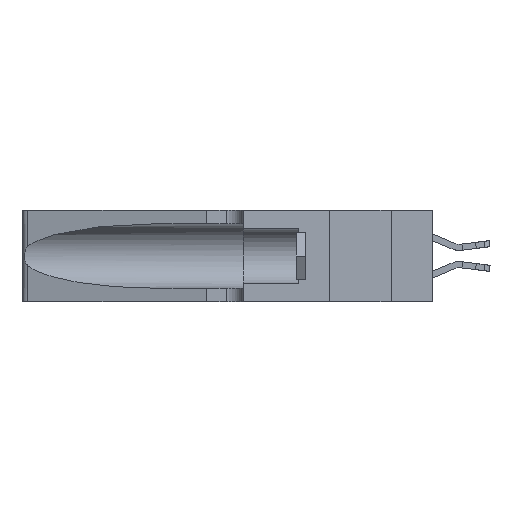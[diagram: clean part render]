
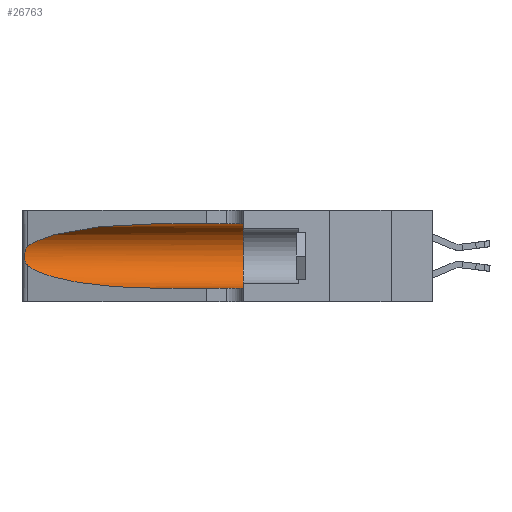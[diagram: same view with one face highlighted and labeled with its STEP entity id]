
A CAD part, left-side view. The second image highlights one B-rep face of the part: STEP entity #26763.
In plain terms, the highlighted cylindrical face has radius 3.308 mm (diameter 6.617 mm), a partial arc.
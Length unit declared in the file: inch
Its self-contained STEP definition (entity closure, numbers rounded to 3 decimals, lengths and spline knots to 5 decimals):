
#620 = ORIENTED_EDGE ( 'NONE', *, *, #31915, .T. ) ;
#2100 = AXIS2_PLACEMENT_3D ( 'NONE', #21576, #31954, #15879 ) ;
#2142 = CARTESIAN_POINT ( 'NONE',  ( 0.1305, 1.61858, 0.05475 ) ) ;
#2274 = CARTESIAN_POINT ( 'NONE',  ( 0.25487, 1.22718, 0.22369 ) ) ;
#3947 = ORIENTED_EDGE ( 'NONE', *, *, #4790, .T. ) ;
#4188 = VERTEX_POINT ( 'NONE', #12258 ) ;
#4305 = CARTESIAN_POINT ( 'NONE',  ( 0.25487, 1.22718, 0.22369 ) ) ;
#4382 = LINE ( 'NONE', #5252, #24743 ) ;
#4790 = EDGE_CURVE ( 'NONE', #32693, #4188, #27645, .T. ) ;
#5252 = CARTESIAN_POINT ( 'NONE',  ( 0.1305, 1.61858, 0.31525 ) ) ;
#5583 = CARTESIAN_POINT ( 'NONE',  ( 0.25639, 1.23186, 0.15144 ) ) ;
#6110 = FACE_OUTER_BOUND ( 'NONE', #24389, .T. ) ;
#7301 = CARTESIAN_POINT ( 'NONE',  ( 0.25555, 1.22994, 0.2215 ) ) ;
#7967 = CARTESIAN_POINT ( 'NONE',  ( 0.26075, 1.23896, 0.178 ) ) ;
#9027 = VERTEX_POINT ( 'NONE', #2274 ) ;
#9104 = CARTESIAN_POINT ( 'NONE',  ( 0.1305, 0.35, 0.31525 ) ) ;
#9212 = VERTEX_POINT ( 'NONE', #16954 ) ;
#10148 = DIRECTION ( 'NONE',  ( 0., -1., 0. ) ) ;
#10149 = CARTESIAN_POINT ( 'NONE',  ( 0.1305, 0.72297, 0.31525 ) ) ;
#12258 = CARTESIAN_POINT ( 'NONE',  ( 0.1305, 0.72297, 0.05475 ) ) ;
#12277 = VECTOR ( 'NONE', #10148, 39.37008 ) ;
#13144 = DIRECTION ( 'NONE',  ( 0., -1., 0. ) ) ;
#13155 = CARTESIAN_POINT ( 'NONE',  ( 0.25487, 1.22718, 0.14631 ) ) ;
#13500 = CARTESIAN_POINT ( 'NONE',  ( 0.25555, 1.22993, 0.14849 ) ) ;
#13598 = CARTESIAN_POINT ( 'NONE',  ( 0.26017, 1.23833, 0.17102 ) ) ;
#14024 = CYLINDRICAL_SURFACE ( 'NONE', #2100, 0.13025 ) ;
#15007 = CARTESIAN_POINT ( 'NONE',  ( 0.18966, 0.96281, 0.05475 ) ) ;
#15396 = ORIENTED_EDGE ( 'NONE', *, *, #24523, .T. ) ;
#15879 = DIRECTION ( 'NONE',  ( 0., 0., -1. ) ) ;
#15943 = CARTESIAN_POINT ( 'NONE',  ( 0.26018, 1.23835, 0.19895 ) ) ;
#16114 = EDGE_CURVE ( 'NONE', #4188, #17780, #29689, .T. ) ;
#16166 = EDGE_CURVE ( 'NONE', #9212, #17867, #4382, .T. ) ;
#16954 = CARTESIAN_POINT ( 'NONE',  ( 0.1305, 0.72297, 0.31525 ) ) ;
#17100 = CARTESIAN_POINT ( 'NONE',  ( 0.1305, 0.35, 0.05475 ) ) ;
#17201 = CARTESIAN_POINT ( 'NONE',  ( 0.2373, 1.15595, 0.08982 ) ) ;
#17780 = VERTEX_POINT ( 'NONE', #17100 ) ;
#17867 = VERTEX_POINT ( 'NONE', #9104 ) ;
#18138 = DIRECTION ( 'NONE',  ( 0., 1., 0. ) ) ;
#18694 = CARTESIAN_POINT ( 'NONE',  ( 0.25487, 1.22718, 0.14631 ) ) ;
#20263 = CARTESIAN_POINT ( 'NONE',  ( 0.1305, 0.72297, 0.05475 ) ) ;
#20364 = CARTESIAN_POINT ( 'NONE',  ( 0.2373, 1.15595, 0.28018 ) ) ;
#20965 = CARTESIAN_POINT ( 'NONE',  ( 0.25787, 1.23484, 0.2124 ) ) ;
#21195 = CARTESIAN_POINT ( 'NONE',  ( 0.25856, 1.23593, 0.16098 ) ) ;
#21275 = AXIS2_PLACEMENT_3D ( 'NONE', #23630, #18138, #31538 ) ;
#21314 = CARTESIAN_POINT ( 'NONE',  ( 0.25789, 1.23486, 0.15765 ) ) ;
#21576 = CARTESIAN_POINT ( 'NONE',  ( 0.1305, 1.61858, 0.185 ) ) ;
#23243 = B_SPLINE_CURVE_WITH_KNOTS ( 'NONE', 3,
 ( #23566, #7301, #28868, #20965, #25879, #15943, #29504, #7967, #13598, #21195, #21314, #5583, #13500, #13155 ),
 .UNSPECIFIED., .F., .F.,
 ( 4, 2, 2, 2, 2, 2, 4 ),
 ( 0., 0.00027, 0.00053, 0.00107, 0.0016, 0.00187, 0.00214 ),
 .UNSPECIFIED. ) ;
#23566 = CARTESIAN_POINT ( 'NONE',  ( 0.25487, 1.22718, 0.22369 ) ) ;
#23630 = CARTESIAN_POINT ( 'NONE',  ( 0.1305, 0.35, 0.185 ) ) ;
#24389 = EDGE_LOOP ( 'NONE', ( #15396, #620, #3947, #33166, #31539, #25721 ) ) ;
#24523 = EDGE_CURVE ( 'NONE', #9212, #9027, #31443, .T. ) ;
#24743 = VECTOR ( 'NONE', #13144, 39.37008 ) ;
#25368 = CARTESIAN_POINT ( 'NONE',  ( 0.25487, 1.22718, 0.14631 ) ) ;
#25721 = ORIENTED_EDGE ( 'NONE', *, *, #16166, .F. ) ;
#25806 = CIRCLE ( 'NONE', #21275, 0.13025 ) ;
#25879 = CARTESIAN_POINT ( 'NONE',  ( 0.25854, 1.2359, 0.20912 ) ) ;
#26763 = ADVANCED_FACE ( 'NONE', ( #6110 ), #14024, .F. ) ;
#27645 =( BOUNDED_CURVE ( )  B_SPLINE_CURVE ( 3, ( #25368, #17201, #15007, #20263 ),
 .UNSPECIFIED., .F., .T. ) 
 B_SPLINE_CURVE_WITH_KNOTS ( ( 4, 4 ),
 ( 3.44316, 4.71239 ),
 .UNSPECIFIED. ) 
 CURVE ( )  GEOMETRIC_REPRESENTATION_ITEM ( )  RATIONAL_B_SPLINE_CURVE ( ( 1., 0.87, 0.87, 1. ) ) 
 REPRESENTATION_ITEM ( '' )  );
#28868 = CARTESIAN_POINT ( 'NONE',  ( 0.25639, 1.23184, 0.21858 ) ) ;
#29504 = CARTESIAN_POINT ( 'NONE',  ( 0.26075, 1.23896, 0.19203 ) ) ;
#29689 = LINE ( 'NONE', #2142, #12277 ) ;
#30774 = CARTESIAN_POINT ( 'NONE',  ( 0.18966, 0.96281, 0.31525 ) ) ;
#31443 =( BOUNDED_CURVE ( )  B_SPLINE_CURVE ( 3, ( #10149, #30774, #20364, #4305 ),
 .UNSPECIFIED., .F., .T. ) 
 B_SPLINE_CURVE_WITH_KNOTS ( ( 4, 4 ),
 ( 1.5708, 2.84003 ),
 .UNSPECIFIED. ) 
 CURVE ( )  GEOMETRIC_REPRESENTATION_ITEM ( )  RATIONAL_B_SPLINE_CURVE ( ( 1., 0.87, 0.87, 1. ) ) 
 REPRESENTATION_ITEM ( '' )  );
#31538 = DIRECTION ( 'NONE',  ( 0., 0., 1. ) ) ;
#31539 = ORIENTED_EDGE ( 'NONE', *, *, #32562, .F. ) ;
#31915 = EDGE_CURVE ( 'NONE', #9027, #32693, #23243, .T. ) ;
#31954 = DIRECTION ( 'NONE',  ( 0., -1., 0. ) ) ;
#32562 = EDGE_CURVE ( 'NONE', #17867, #17780, #25806, .T. ) ;
#32693 = VERTEX_POINT ( 'NONE', #18694 ) ;
#33166 = ORIENTED_EDGE ( 'NONE', *, *, #16114, .T. ) ;
